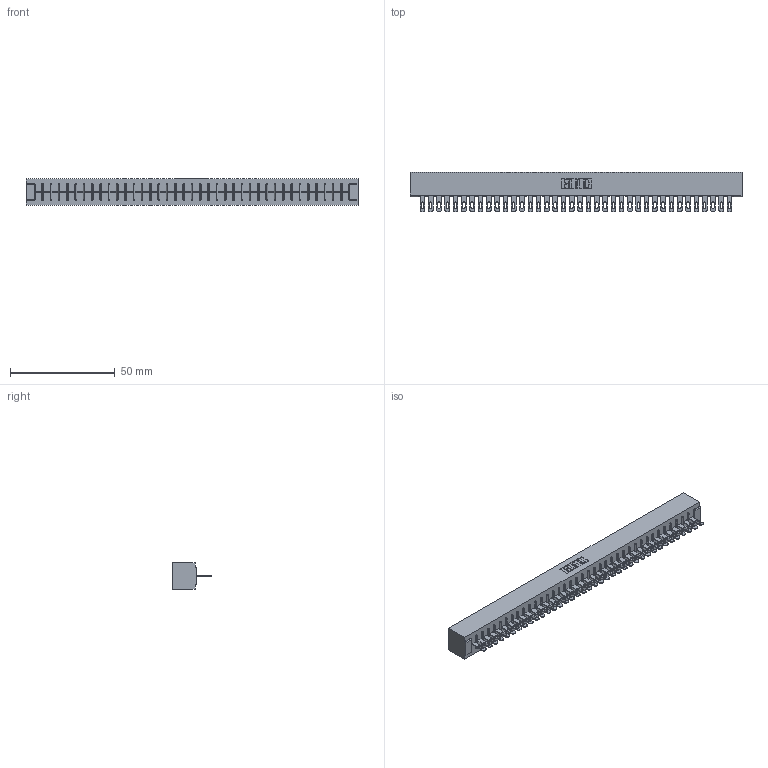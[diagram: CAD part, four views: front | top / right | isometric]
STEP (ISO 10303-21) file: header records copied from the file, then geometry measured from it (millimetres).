
FILE_DESCRIPTION (( 'STEP AP203' ), '1' );
FILE_NAME ('356-038-400-101.STEP', '2020-09-23T23:29:32', ( '' ), ( '' ), 'SwSTEP 2.0', 'SolidWorks 2020', '' );
FILE_SCHEMA (( 'CONFIG_CONTROL_DESIGN' ));
Length unit declared in the file: inch
Products named in the file (3): 356-038-400-101; 306 Part_No Mounting; 306-290-001_100
Assembly tree (39 placements, depth 2):
  356-038-400-101
    306 Part_No Mounting
    306-290-001_100  x38
Bounding box: 158.45 x 18.87 x 12.7 mm (x, y, z)
Volume: 18186.8 mm3; surface area: 19437.1 mm2
Topology: 39 solids, 39 shells, 2996 faces, 8462 edges, 5436 vertices
Faces by surface type: plane 1964, cylinder 880, sphere 152
Entity records: 35841 total; most frequent: CARTESIAN_POINT 6017, ORIENTED_EDGE 5964, DIRECTION 5934, EDGE_CURVE 2982, LINE 2332, VECTOR 2332, VERTEX_POINT 1884, AXIS2_PLACEMENT_3D 1801
